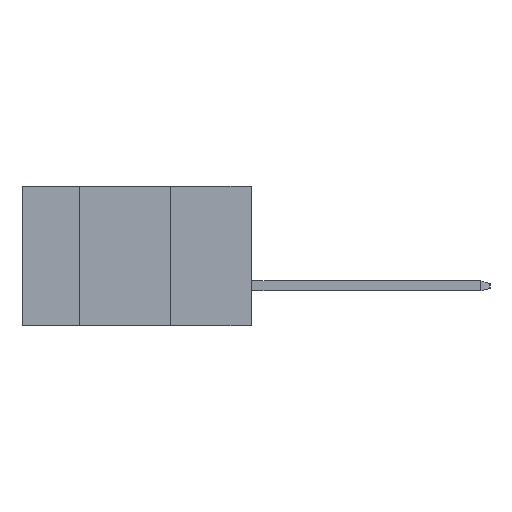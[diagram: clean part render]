
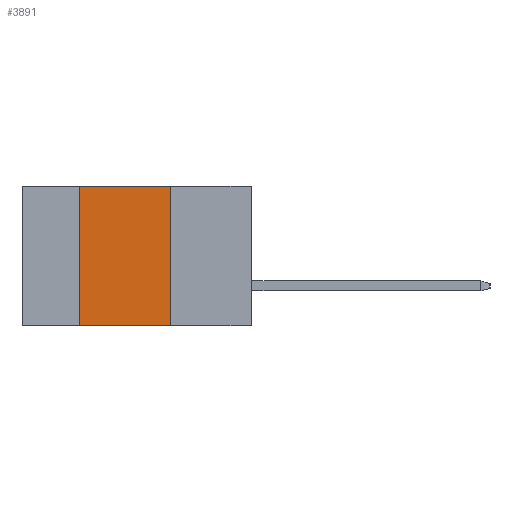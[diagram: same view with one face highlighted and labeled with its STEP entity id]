
A CAD part, left-side view. The second image highlights one B-rep face of the part: STEP entity #3891.
In plain terms, the highlighted planar face has unit normal (-1, 0, 0).
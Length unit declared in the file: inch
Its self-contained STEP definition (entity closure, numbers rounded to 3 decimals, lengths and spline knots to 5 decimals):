
#204 = CARTESIAN_POINT ( 'NONE',  ( 0., 0.54, -0.437 ) ) ;
#457 = EDGE_CURVE ( 'NONE', #3543, #11342, #9251, .T. ) ;
#499 = DIRECTION ( 'NONE',  ( 0., -1., 0. ) ) ;
#1013 = DIRECTION ( 'NONE',  ( 0., 0., -1. ) ) ;
#1048 = EDGE_LOOP ( 'NONE', ( #4119, #8049, #9158, #12512 ) ) ;
#1296 = DIRECTION ( 'NONE',  ( 0., 0., 1. ) ) ;
#1484 = CARTESIAN_POINT ( 'NONE',  ( 0., 0.72, 0. ) ) ;
#1815 = DIRECTION ( 'NONE',  ( 0., -1., 0. ) ) ;
#2520 = CARTESIAN_POINT ( 'NONE',  ( 0., 0.72, -0.437 ) ) ;
#2555 = CARTESIAN_POINT ( 'NONE',  ( 0., 0.54, -0.437 ) ) ;
#3130 = CARTESIAN_POINT ( 'NONE',  ( 0., 0.254, 0. ) ) ;
#3383 = VECTOR ( 'NONE', #1815, 39.37008 ) ;
#3543 = VERTEX_POINT ( 'NONE', #4033 ) ;
#3582 = AXIS2_PLACEMENT_3D ( 'NONE', #1484, #4469, #12267 ) ;
#3803 = VERTEX_POINT ( 'NONE', #2555 ) ;
#3856 = VECTOR ( 'NONE', #1296, 39.37008 ) ;
#3891 = ADVANCED_FACE ( 'NONE', ( #6324 ), #10236, .F. ) ;
#3946 = LINE ( 'NONE', #9760, #11055 ) ;
#4033 = CARTESIAN_POINT ( 'NONE',  ( 0., 0.54, 0. ) ) ;
#4119 = ORIENTED_EDGE ( 'NONE', *, *, #6742, .F. ) ;
#4469 = DIRECTION ( 'NONE',  ( 1., 0., 0. ) ) ;
#4936 = LINE ( 'NONE', #204, #3856 ) ;
#5914 = EDGE_CURVE ( 'NONE', #3803, #11094, #11263, .T. ) ;
#6324 = FACE_OUTER_BOUND ( 'NONE', #1048, .T. ) ;
#6742 = EDGE_CURVE ( 'NONE', #11342, #11094, #3946, .T. ) ;
#7448 = CARTESIAN_POINT ( 'NONE',  ( 0., 0.72, 0. ) ) ;
#8049 = ORIENTED_EDGE ( 'NONE', *, *, #457, .F. ) ;
#9158 = ORIENTED_EDGE ( 'NONE', *, *, #10993, .F. ) ;
#9251 = LINE ( 'NONE', #7448, #9940 ) ;
#9270 = CARTESIAN_POINT ( 'NONE',  ( 0., 0.254, -0.437 ) ) ;
#9760 = CARTESIAN_POINT ( 'NONE',  ( 0., 0.254, -0.437 ) ) ;
#9940 = VECTOR ( 'NONE', #499, 39.37008 ) ;
#10236 = PLANE ( 'NONE',  #3582 ) ;
#10993 = EDGE_CURVE ( 'NONE', #3803, #3543, #4936, .T. ) ;
#11055 = VECTOR ( 'NONE', #1013, 39.37008 ) ;
#11094 = VERTEX_POINT ( 'NONE', #9270 ) ;
#11263 = LINE ( 'NONE', #2520, #3383 ) ;
#11342 = VERTEX_POINT ( 'NONE', #3130 ) ;
#12267 = DIRECTION ( 'NONE',  ( 0., 0., -1. ) ) ;
#12512 = ORIENTED_EDGE ( 'NONE', *, *, #5914, .T. ) ;
